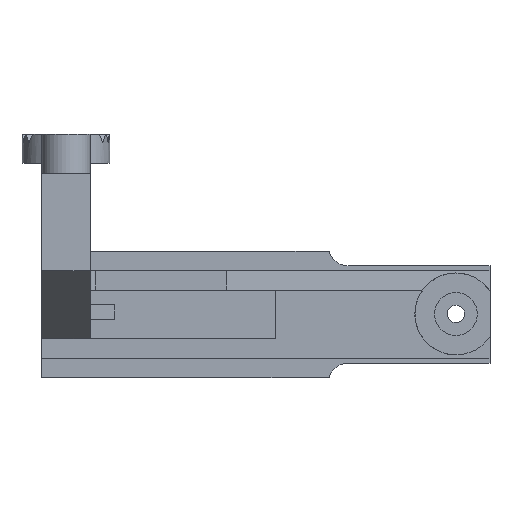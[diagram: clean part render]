
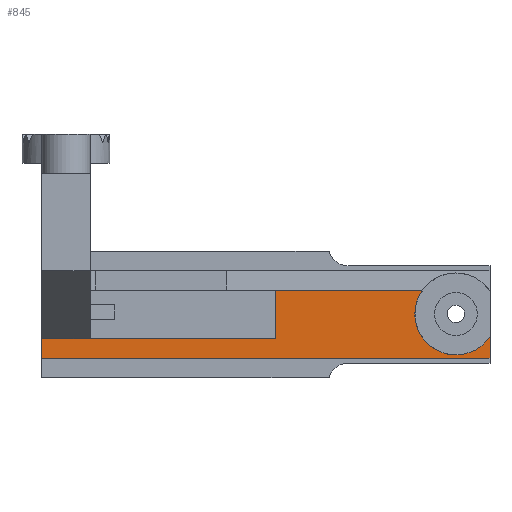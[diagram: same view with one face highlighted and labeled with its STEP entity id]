
A CAD part, front view. The second image highlights one B-rep face of the part: STEP entity #845.
In plain terms, the highlighted planar face has unit normal (0, -1, 0).
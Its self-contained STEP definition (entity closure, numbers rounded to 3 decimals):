
#94 = CIRCLE ( 'NONE', #2697, 4.2 ) ;
#131 = DIRECTION ( 'NONE',  ( 0., 0., -1. ) ) ;
#158 = CARTESIAN_POINT ( 'NONE',  ( -15.586, 11., -19. ) ) ;
#172 = LINE ( 'NONE', #1532, #476 ) ;
#193 = AXIS2_PLACEMENT_3D ( 'NONE', #1873, #2819, #1892 ) ;
#223 = LINE ( 'NONE', #1611, #849 ) ;
#277 = VECTOR ( 'NONE', #131, 1000. ) ;
#340 = CARTESIAN_POINT ( 'NONE',  ( -2.5, 11., -17. ) ) ;
#405 = CIRCLE ( 'NONE', #193, 4.2 ) ;
#422 = DIRECTION ( 'NONE',  ( 1., 0., 0. ) ) ;
#476 = VECTOR ( 'NONE', #1021, 1000. ) ;
#551 = ORIENTED_EDGE ( 'NONE', *, *, #2545, .T. ) ;
#566 = DIRECTION ( 'NONE',  ( 0., 0., -1. ) ) ;
#593 = ORIENTED_EDGE ( 'NONE', *, *, #2430, .F. ) ;
#638 = CARTESIAN_POINT ( 'NONE',  ( 43.5, 11., -19. ) ) ;
#749 = CARTESIAN_POINT ( 'NONE',  ( 21.5, 11., -12. ) ) ;
#760 = AXIS2_PLACEMENT_3D ( 'NONE', #955, #1678, #2648 ) ;
#782 = EDGE_CURVE ( 'NONE', #2025, #2689, #1390, .T. ) ;
#801 = VECTOR ( 'NONE', #853, 1000. ) ;
#845 = ADVANCED_FACE ( 'NONE', ( #2439 ), #3135, .T. ) ;
#849 = VECTOR ( 'NONE', #1144, 1000. ) ;
#853 = DIRECTION ( 'NONE',  ( 1., 0., 0. ) ) ;
#886 = ORIENTED_EDGE ( 'NONE', *, *, #1001, .F. ) ;
#955 = CARTESIAN_POINT ( 'NONE',  ( -15.586, 11., -10. ) ) ;
#957 = CARTESIAN_POINT ( 'NONE',  ( 36.584, 11., -12. ) ) ;
#1001 = EDGE_CURVE ( 'NONE', #1663, #2417, #223, .T. ) ;
#1005 = ORIENTED_EDGE ( 'NONE', *, *, #782, .F. ) ;
#1016 = VERTEX_POINT ( 'NONE', #1215 ) ;
#1021 = DIRECTION ( 'NONE',  ( -1., 0., 0. ) ) ;
#1144 = DIRECTION ( 'NONE',  ( 0., 0., 1. ) ) ;
#1146 = CARTESIAN_POINT ( 'NONE',  ( 0., 11., -12. ) ) ;
#1208 = CARTESIAN_POINT ( 'NONE',  ( -2.5, 11., -19. ) ) ;
#1215 = CARTESIAN_POINT ( 'NONE',  ( 21.5, 11., -17. ) ) ;
#1219 = CARTESIAN_POINT ( 'NONE',  ( 21.5, 11., -12. ) ) ;
#1256 = EDGE_CURVE ( 'NONE', #2689, #1868, #94, .T. ) ;
#1264 = LINE ( 'NONE', #158, #801 ) ;
#1302 = VERTEX_POINT ( 'NONE', #1310 ) ;
#1310 = CARTESIAN_POINT ( 'NONE',  ( 43.5, 11., -16.765 ) ) ;
#1332 = EDGE_CURVE ( 'NONE', #1868, #1302, #405, .T. ) ;
#1390 = LINE ( 'NONE', #1146, #3065 ) ;
#1416 = VERTEX_POINT ( 'NONE', #638 ) ;
#1418 = ORIENTED_EDGE ( 'NONE', *, *, #1332, .F. ) ;
#1485 = ORIENTED_EDGE ( 'NONE', *, *, #2839, .T. ) ;
#1508 = EDGE_LOOP ( 'NONE', ( #593, #1418, #1989, #1005, #2535, #1485, #886, #551 ) ) ;
#1532 = CARTESIAN_POINT ( 'NONE',  ( 23.651, 11., -17. ) ) ;
#1611 = CARTESIAN_POINT ( 'NONE',  ( -2.5, 11., -10. ) ) ;
#1663 = VERTEX_POINT ( 'NONE', #1208 ) ;
#1678 = DIRECTION ( 'NONE',  ( 0., -1., 0. ) ) ;
#1758 = DIRECTION ( 'NONE',  ( 0., 0., 1. ) ) ;
#1868 = VERTEX_POINT ( 'NONE', #2148 ) ;
#1873 = CARTESIAN_POINT ( 'NONE',  ( 40., 11., -14.443 ) ) ;
#1892 = DIRECTION ( 'NONE',  ( 0., 0., -1. ) ) ;
#1989 = ORIENTED_EDGE ( 'NONE', *, *, #1256, .F. ) ;
#2025 = VERTEX_POINT ( 'NONE', #1219 ) ;
#2044 = DIRECTION ( 'NONE',  ( 0., -1., 0. ) ) ;
#2079 = EDGE_CURVE ( 'NONE', #1016, #2025, #2366, .T. ) ;
#2129 = CARTESIAN_POINT ( 'NONE',  ( 43.5, 11., -10. ) ) ;
#2148 = CARTESIAN_POINT ( 'NONE',  ( 40., 11., -18.643 ) ) ;
#2366 = LINE ( 'NONE', #749, #2955 ) ;
#2417 = VERTEX_POINT ( 'NONE', #340 ) ;
#2430 = EDGE_CURVE ( 'NONE', #1302, #1416, #2885, .T. ) ;
#2439 = FACE_OUTER_BOUND ( 'NONE', #1508, .T. ) ;
#2535 = ORIENTED_EDGE ( 'NONE', *, *, #2079, .F. ) ;
#2545 = EDGE_CURVE ( 'NONE', #1663, #1416, #1264, .T. ) ;
#2648 = DIRECTION ( 'NONE',  ( 0., 0., -1. ) ) ;
#2689 = VERTEX_POINT ( 'NONE', #957 ) ;
#2697 = AXIS2_PLACEMENT_3D ( 'NONE', #3014, #2044, #566 ) ;
#2819 = DIRECTION ( 'NONE',  ( 0., -1., 0. ) ) ;
#2839 = EDGE_CURVE ( 'NONE', #1016, #2417, #172, .T. ) ;
#2885 = LINE ( 'NONE', #2129, #277 ) ;
#2955 = VECTOR ( 'NONE', #1758, 1000. ) ;
#3014 = CARTESIAN_POINT ( 'NONE',  ( 40., 11., -14.443 ) ) ;
#3065 = VECTOR ( 'NONE', #422, 1000. ) ;
#3135 = PLANE ( 'NONE',  #760 ) ;
